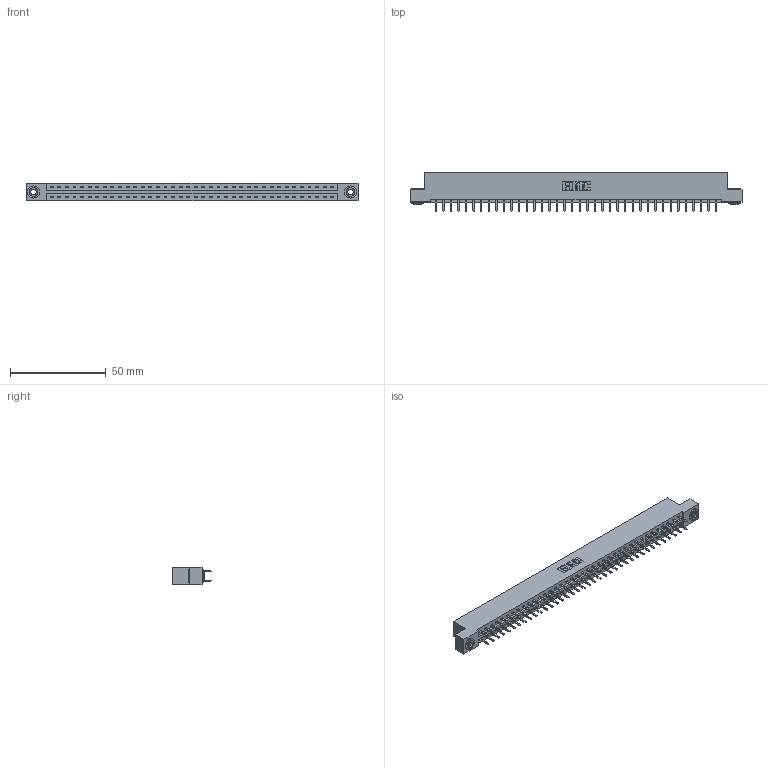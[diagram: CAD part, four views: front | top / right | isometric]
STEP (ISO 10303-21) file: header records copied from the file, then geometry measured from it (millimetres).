
FILE_DESCRIPTION (( 'STEP AP203' ), '1' );
FILE_NAME ('387-076-520-203.STEP', '2018-09-22T20:54:36', ( '' ), ( '' ), 'SwSTEP 2.0', 'SolidWorks 2016', '' );
FILE_SCHEMA (( 'CONFIG_CONTROL_DESIGN' ));
Length unit declared in the file: inch
Products named in the file (4): 345-292-001_345-293-120; 345-250-002_345-250-002-102; 387-076-520-203; 337 Part_Flush Mounting Lugs - 0.156 Dia-TH
Assembly tree (79 placements, depth 2):
  387-076-520-203
    337 Part_Flush Mounting Lugs - 0.156 Dia-TH
    345-292-001_345-293-120  x76
    345-250-002_345-250-002-102  x2
Bounding box: 173.58 x 20.02 x 9.4 mm (x, y, z)
Volume: 18226.4 mm3; surface area: 20695.2 mm2
Topology: 79 solids, 79 shells, 4560 faces, 13231 edges, 8614 vertices
Faces by surface type: plane 3120, cylinder 1432, cone 8
Entity records: 30744 total; most frequent: CARTESIAN_POINT 5169, ORIENTED_EDGE 5086, DIRECTION 4425, EDGE_CURVE 2543, LINE 2387, VECTOR 2387, VERTEX_POINT 1690, AXIS2_PLACEMENT_3D 1019
